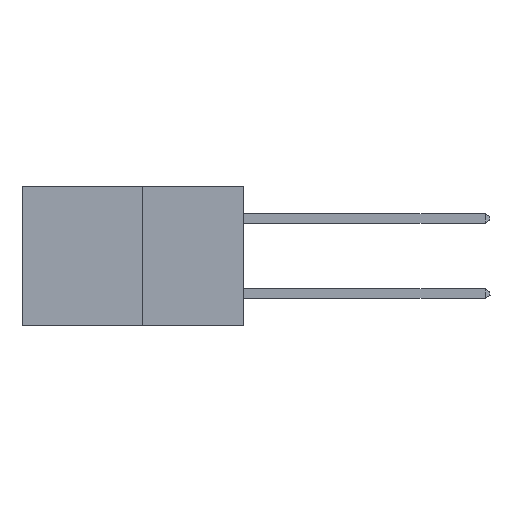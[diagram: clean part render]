
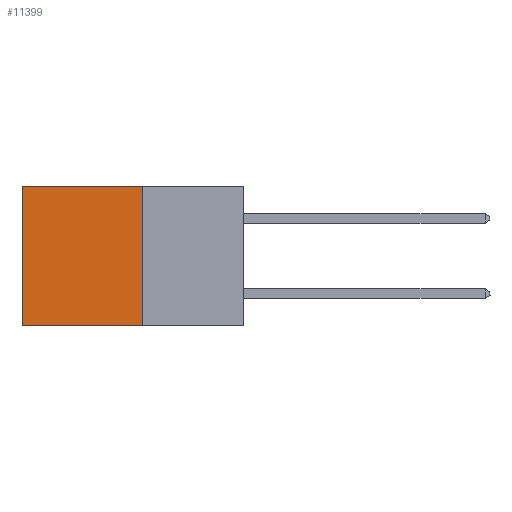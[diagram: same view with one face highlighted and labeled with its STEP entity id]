
A CAD part, left-side view. The second image highlights one B-rep face of the part: STEP entity #11399.
In plain terms, the highlighted planar face has unit normal (-1, 0, 0).
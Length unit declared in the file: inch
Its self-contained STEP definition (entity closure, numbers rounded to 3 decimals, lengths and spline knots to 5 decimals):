
#552 = VECTOR ( 'NONE', #25724, 39.37008 ) ;
#1317 = CARTESIAN_POINT ( 'NONE',  ( 0.277, 0.27, -0.37 ) ) ;
#2330 = EDGE_CURVE ( 'NONE', #23115, #15197, #5841, .T. ) ;
#2403 = EDGE_LOOP ( 'NONE', ( #15892, #5825, #22249, #4802 ) ) ;
#2595 = VECTOR ( 'NONE', #12249, 39.37008 ) ;
#3674 = EDGE_CURVE ( 'NONE', #15127, #5543, #5759, .T. ) ;
#4005 = EDGE_CURVE ( 'NONE', #23115, #15127, #26264, .T. ) ;
#4802 = ORIENTED_EDGE ( 'NONE', *, *, #2330, .T. ) ;
#5543 = VERTEX_POINT ( 'NONE', #19513 ) ;
#5759 = LINE ( 'NONE', #25912, #552 ) ;
#5825 = ORIENTED_EDGE ( 'NONE', *, *, #3674, .F. ) ;
#5841 = LINE ( 'NONE', #22239, #18508 ) ;
#8077 = DIRECTION ( 'NONE',  ( 0., 0., -1. ) ) ;
#9222 = FACE_OUTER_BOUND ( 'NONE', #2403, .T. ) ;
#9262 = LINE ( 'NONE', #12405, #25689 ) ;
#11399 = ADVANCED_FACE ( 'NONE', ( #9222 ), #18965, .F. ) ;
#12249 = DIRECTION ( 'NONE',  ( 0., 0., -1. ) ) ;
#12405 = CARTESIAN_POINT ( 'NONE',  ( 0.277, 0.59, -0.37 ) ) ;
#12554 = CARTESIAN_POINT ( 'NONE',  ( 0.277, 0.27, -0.37 ) ) ;
#13900 = CARTESIAN_POINT ( 'NONE',  ( 0.277, 0.27, -0.37 ) ) ;
#14720 = DIRECTION ( 'NONE',  ( 0., 0., -1. ) ) ;
#15127 = VERTEX_POINT ( 'NONE', #13900 ) ;
#15197 = VERTEX_POINT ( 'NONE', #26922 ) ;
#15892 = ORIENTED_EDGE ( 'NONE', *, *, #26723, .T. ) ;
#17196 = CARTESIAN_POINT ( 'NONE',  ( 0.277, 0.27, 0. ) ) ;
#18223 = DIRECTION ( 'NONE',  ( 0., 1., 0. ) ) ;
#18508 = VECTOR ( 'NONE', #18223, 39.37008 ) ;
#18965 = PLANE ( 'NONE',  #23686 ) ;
#19513 = CARTESIAN_POINT ( 'NONE',  ( 0.277, 0.59, -0.37 ) ) ;
#22239 = CARTESIAN_POINT ( 'NONE',  ( 0.277, 0.27, 0. ) ) ;
#22249 = ORIENTED_EDGE ( 'NONE', *, *, #4005, .F. ) ;
#23115 = VERTEX_POINT ( 'NONE', #17196 ) ;
#23686 = AXIS2_PLACEMENT_3D ( 'NONE', #12554, #27502, #14720 ) ;
#25689 = VECTOR ( 'NONE', #8077, 39.37008 ) ;
#25724 = DIRECTION ( 'NONE',  ( 0., 1., 0. ) ) ;
#25912 = CARTESIAN_POINT ( 'NONE',  ( 0.277, 0.27, -0.37 ) ) ;
#26264 = LINE ( 'NONE', #1317, #2595 ) ;
#26723 = EDGE_CURVE ( 'NONE', #15197, #5543, #9262, .T. ) ;
#26922 = CARTESIAN_POINT ( 'NONE',  ( 0.277, 0.59, 0. ) ) ;
#27502 = DIRECTION ( 'NONE',  ( 1., 0., 0. ) ) ;
